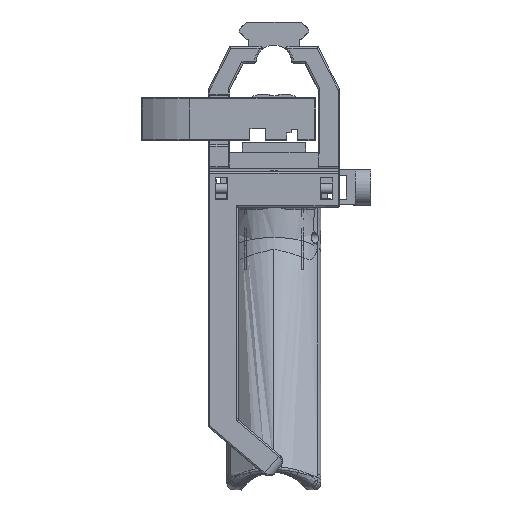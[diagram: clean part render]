
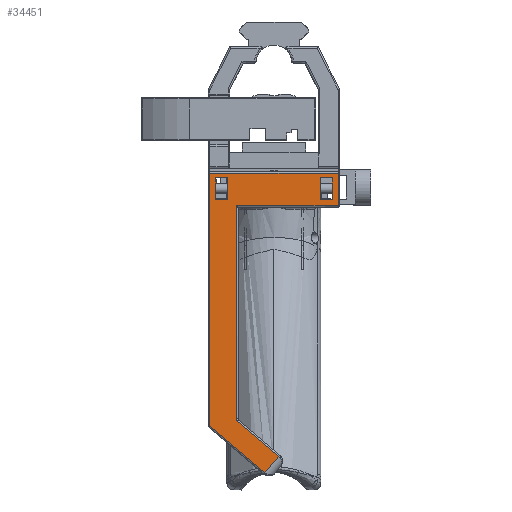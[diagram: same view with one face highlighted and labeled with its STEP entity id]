
A CAD part, left-side view. The second image highlights one B-rep face of the part: STEP entity #34451.
In plain terms, the highlighted planar face has unit normal (-1, 0, 0).
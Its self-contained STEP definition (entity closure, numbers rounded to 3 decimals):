
#325=FACE_BOUND('',#6641,.T.);
#326=FACE_BOUND('',#6642,.T.);
#1144=CIRCLE('',#37151,1.);
#4729=FACE_OUTER_BOUND('',#6640,.T.);
#6640=EDGE_LOOP('',(#30748,#30749,#30750,#30751,#30752,#30753,#30754,#30755,
#30756));
#6641=EDGE_LOOP('',(#30757,#30758,#30759,#30760));
#6642=EDGE_LOOP('',(#30761,#30762,#30763,#30764));
#9358=LINE('',#89738,#12171);
#9362=LINE('',#89759,#12175);
#9363=LINE('',#89763,#12176);
#9364=LINE('',#89765,#12177);
#9365=LINE('',#89767,#12178);
#9366=LINE('',#89769,#12179);
#9367=LINE('',#89773,#12180);
#9368=LINE('',#89774,#12181);
#9369=LINE('',#89777,#12182);
#9370=LINE('',#89779,#12183);
#9371=LINE('',#89781,#12184);
#9372=LINE('',#89782,#12185);
#9373=LINE('',#89785,#12186);
#9374=LINE('',#89787,#12187);
#9375=LINE('',#89789,#12188);
#9376=LINE('',#89790,#12189);
#12171=VECTOR('',#44797,10.);
#12175=VECTOR('',#44827,10.);
#12176=VECTOR('',#44832,0.5);
#12177=VECTOR('',#44833,10.);
#12178=VECTOR('',#44834,10.);
#12179=VECTOR('',#44835,10.);
#12180=VECTOR('',#44838,10.);
#12181=VECTOR('',#44839,10.);
#12182=VECTOR('',#44840,10.);
#12183=VECTOR('',#44841,10.);
#12184=VECTOR('',#44842,10.);
#12185=VECTOR('',#44843,10.);
#12186=VECTOR('',#44844,10.);
#12187=VECTOR('',#44845,10.);
#12188=VECTOR('',#44846,10.);
#12189=VECTOR('',#44847,10.);
#15961=VERTEX_POINT('',#89733);
#15962=VERTEX_POINT('',#89736);
#15966=VERTEX_POINT('',#89758);
#15967=VERTEX_POINT('',#89762);
#15968=VERTEX_POINT('',#89764);
#15969=VERTEX_POINT('',#89766);
#15970=VERTEX_POINT('',#89768);
#15971=VERTEX_POINT('',#89770);
#15972=VERTEX_POINT('',#89772);
#15973=VERTEX_POINT('',#89775);
#15974=VERTEX_POINT('',#89776);
#15975=VERTEX_POINT('',#89778);
#15976=VERTEX_POINT('',#89780);
#15977=VERTEX_POINT('',#89783);
#15978=VERTEX_POINT('',#89784);
#15979=VERTEX_POINT('',#89786);
#15980=VERTEX_POINT('',#89788);
#20936=EDGE_CURVE('',#15962,#15961,#9358,.T.);
#20946=EDGE_CURVE('',#15961,#15966,#9362,.T.);
#20948=EDGE_CURVE('',#15967,#15962,#9363,.T.);
#20949=EDGE_CURVE('',#15968,#15967,#9364,.T.);
#20950=EDGE_CURVE('',#15969,#15968,#9365,.T.);
#20951=EDGE_CURVE('',#15970,#15969,#9366,.T.);
#20952=EDGE_CURVE('',#15971,#15970,#1144,.T.);
#20953=EDGE_CURVE('',#15972,#15971,#9367,.T.);
#20954=EDGE_CURVE('',#15966,#15972,#9368,.T.);
#20955=EDGE_CURVE('',#15973,#15974,#9369,.T.);
#20956=EDGE_CURVE('',#15974,#15975,#9370,.T.);
#20957=EDGE_CURVE('',#15975,#15976,#9371,.T.);
#20958=EDGE_CURVE('',#15976,#15973,#9372,.T.);
#20959=EDGE_CURVE('',#15977,#15978,#9373,.T.);
#20960=EDGE_CURVE('',#15978,#15979,#9374,.T.);
#20961=EDGE_CURVE('',#15979,#15980,#9375,.T.);
#20962=EDGE_CURVE('',#15980,#15977,#9376,.T.);
#30748=ORIENTED_EDGE('',*,*,#20936,.F.);
#30749=ORIENTED_EDGE('',*,*,#20948,.F.);
#30750=ORIENTED_EDGE('',*,*,#20949,.F.);
#30751=ORIENTED_EDGE('',*,*,#20950,.F.);
#30752=ORIENTED_EDGE('',*,*,#20951,.F.);
#30753=ORIENTED_EDGE('',*,*,#20952,.F.);
#30754=ORIENTED_EDGE('',*,*,#20953,.F.);
#30755=ORIENTED_EDGE('',*,*,#20954,.F.);
#30756=ORIENTED_EDGE('',*,*,#20946,.F.);
#30757=ORIENTED_EDGE('',*,*,#20955,.T.);
#30758=ORIENTED_EDGE('',*,*,#20956,.T.);
#30759=ORIENTED_EDGE('',*,*,#20957,.T.);
#30760=ORIENTED_EDGE('',*,*,#20958,.T.);
#30761=ORIENTED_EDGE('',*,*,#20959,.T.);
#30762=ORIENTED_EDGE('',*,*,#20960,.T.);
#30763=ORIENTED_EDGE('',*,*,#20961,.T.);
#30764=ORIENTED_EDGE('',*,*,#20962,.T.);
#32721=PLANE('',#37150);
#34451=ADVANCED_FACE('',(#4729,#325,#326),#32721,.T.);
#37150=AXIS2_PLACEMENT_3D('',#89761,#44830,#44831);
#37151=AXIS2_PLACEMENT_3D('',#89771,#44836,#44837);
#44797=DIRECTION('',(0.,0.,1.));
#44827=DIRECTION('',(0.,-1.,0.));
#44830=DIRECTION('center_axis',(-1.,0.,0.));
#44831=DIRECTION('ref_axis',(0.,0.,1.));
#44832=DIRECTION('',(0.,1.,0.));
#44833=DIRECTION('',(0.,0.649,-0.76));
#44834=DIRECTION('',(0.,-0.76,-0.649));
#44835=DIRECTION('',(0.,-0.649,0.76));
#44836=DIRECTION('center_axis',(-1.,0.,0.));
#44837=DIRECTION('ref_axis',(0.,-0.419,-0.908));
#44838=DIRECTION('',(0.,-1.,0.));
#44839=DIRECTION('',(0.,0.,-1.));
#44840=DIRECTION('',(0.,0.,-1.));
#44841=DIRECTION('',(0.,1.,0.));
#44842=DIRECTION('',(0.,0.,1.));
#44843=DIRECTION('',(0.,-1.,0.));
#44844=DIRECTION('',(0.,0.,1.));
#44845=DIRECTION('',(0.,-1.,0.));
#44846=DIRECTION('',(0.,0.,-1.));
#44847=DIRECTION('',(0.,1.,0.));
#89733=CARTESIAN_POINT('',(56.755,58.181,19.663));
#89736=CARTESIAN_POINT('',(56.755,58.181,-19.662));
#89738=CARTESIAN_POINT('',(56.755,58.181,2.973));
#89758=CARTESIAN_POINT('',(56.755,48.345,19.663));
#89759=CARTESIAN_POINT('',(56.755,50.429,19.663));
#89761=CARTESIAN_POINT('Origin',(56.755,53.513,-4.515));
#89762=CARTESIAN_POINT('',(56.755,-19.106,-19.662));
#89763=CARTESIAN_POINT('',(56.755,56.597,-19.662));
#89764=CARTESIAN_POINT('',(56.755,-33.499,-2.806));
#89765=CARTESIAN_POINT('',(56.755,-9.273,-31.178));
#89766=CARTESIAN_POINT('',(56.755,-28.496,1.466));
#89767=CARTESIAN_POINT('',(56.755,-3.624,22.704));
#89768=CARTESIAN_POINT('',(56.755,-17.728,-11.145));
#89769=CARTESIAN_POINT('',(56.755,-4.27,-26.906));
#89770=CARTESIAN_POINT('',(56.755,-16.967,-11.495));
#89771=CARTESIAN_POINT('Origin',(56.755,-16.967,-10.495));
#89772=CARTESIAN_POINT('',(56.755,48.345,-11.495));
#89773=CARTESIAN_POINT('',(56.755,50.429,-11.495));
#89774=CARTESIAN_POINT('',(56.755,48.345,-12.004));
#89775=CARTESIAN_POINT('',(56.755,50.246,-14.1));
#89776=CARTESIAN_POINT('',(56.755,50.246,-17.781));
#89777=CARTESIAN_POINT('',(56.755,50.246,-11.048));
#89778=CARTESIAN_POINT('',(56.755,56.801,-17.781));
#89779=CARTESIAN_POINT('',(56.755,55.107,-17.781));
#89780=CARTESIAN_POINT('',(56.755,56.801,-14.1));
#89781=CARTESIAN_POINT('',(56.755,56.801,-9.208));
#89782=CARTESIAN_POINT('',(56.755,51.929,-14.1));
#89783=CARTESIAN_POINT('',(56.755,56.801,14.102));
#89784=CARTESIAN_POINT('',(56.755,56.801,17.782));
#89785=CARTESIAN_POINT('',(56.755,56.801,6.534));
#89786=CARTESIAN_POINT('',(56.755,50.246,17.782));
#89787=CARTESIAN_POINT('',(56.755,51.929,17.782));
#89788=CARTESIAN_POINT('',(56.755,50.246,14.102));
#89789=CARTESIAN_POINT('',(56.755,50.246,4.693));
#89790=CARTESIAN_POINT('',(56.755,55.107,14.102));
